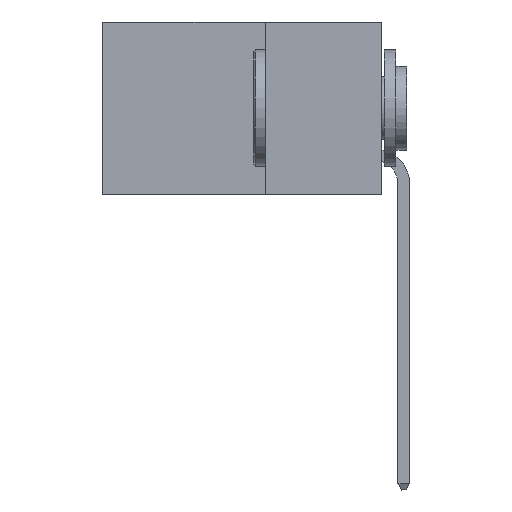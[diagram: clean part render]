
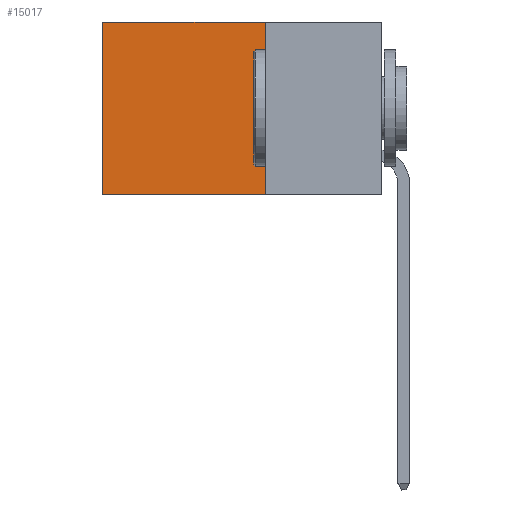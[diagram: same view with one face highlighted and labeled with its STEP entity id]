
A CAD part, left-side view. The second image highlights one B-rep face of the part: STEP entity #15017.
In plain terms, the highlighted planar face has unit normal (-1, 0, 0).
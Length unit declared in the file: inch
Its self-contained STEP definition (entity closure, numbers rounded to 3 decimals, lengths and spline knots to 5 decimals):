
#674 = LINE ( 'NONE', #44026, #37747 ) ;
#1916 = EDGE_LOOP ( 'NONE', ( #40481, #41834, #44903, #2438 ) ) ;
#2438 = ORIENTED_EDGE ( 'NONE', *, *, #30803, .T. ) ;
#5627 = DIRECTION ( 'NONE',  ( 0., 0., -1. ) ) ;
#7217 = EDGE_CURVE ( 'NONE', #43208, #20553, #37806, .T. ) ;
#10774 = VECTOR ( 'NONE', #5627, 39.37008 ) ;
#12456 = EDGE_CURVE ( 'NONE', #20553, #42299, #674, .T. ) ;
#13764 = CARTESIAN_POINT ( 'NONE',  ( 0.2875, 0.25, 0. ) ) ;
#14075 = DIRECTION ( 'NONE',  ( 0., 0., -1. ) ) ;
#14415 = VECTOR ( 'NONE', #17341, 39.37008 ) ;
#14515 = CARTESIAN_POINT ( 'NONE',  ( 0.2875, 0.25, 0. ) ) ;
#14993 = CARTESIAN_POINT ( 'NONE',  ( 0.2875, 0.25, -0.37 ) ) ;
#15017 = ADVANCED_FACE ( 'NONE', ( #31321 ), #45950, .F. ) ;
#17226 = CARTESIAN_POINT ( 'NONE',  ( 0.2875, 0.6, -0.37 ) ) ;
#17341 = DIRECTION ( 'NONE',  ( 0., 1., 0. ) ) ;
#19811 = CARTESIAN_POINT ( 'NONE',  ( 0.2875, 0.25, 0. ) ) ;
#20553 = VERTEX_POINT ( 'NONE', #14993 ) ;
#22053 = CARTESIAN_POINT ( 'NONE',  ( 0.2875, 0.6, 0. ) ) ;
#23967 = LINE ( 'NONE', #24135, #14415 ) ;
#24135 = CARTESIAN_POINT ( 'NONE',  ( 0.2875, 0.25, 0. ) ) ;
#26344 = DIRECTION ( 'NONE',  ( 0., 0., -1. ) ) ;
#29190 = DIRECTION ( 'NONE',  ( 0., 1., 0. ) ) ;
#29609 = EDGE_CURVE ( 'NONE', #32860, #42299, #34507, .T. ) ;
#30803 = EDGE_CURVE ( 'NONE', #43208, #32860, #23967, .T. ) ;
#31039 = AXIS2_PLACEMENT_3D ( 'NONE', #13764, #31911, #14075 ) ;
#31321 = FACE_OUTER_BOUND ( 'NONE', #1916, .T. ) ;
#31911 = DIRECTION ( 'NONE',  ( 1., 0., 0. ) ) ;
#32860 = VERTEX_POINT ( 'NONE', #22053 ) ;
#34507 = LINE ( 'NONE', #44476, #46339 ) ;
#37747 = VECTOR ( 'NONE', #29190, 39.37008 ) ;
#37806 = LINE ( 'NONE', #19811, #10774 ) ;
#40481 = ORIENTED_EDGE ( 'NONE', *, *, #29609, .T. ) ;
#41834 = ORIENTED_EDGE ( 'NONE', *, *, #12456, .F. ) ;
#42299 = VERTEX_POINT ( 'NONE', #17226 ) ;
#43208 = VERTEX_POINT ( 'NONE', #14515 ) ;
#44026 = CARTESIAN_POINT ( 'NONE',  ( 0.2875, 0.25, -0.37 ) ) ;
#44476 = CARTESIAN_POINT ( 'NONE',  ( 0.2875, 0.6, 0. ) ) ;
#44903 = ORIENTED_EDGE ( 'NONE', *, *, #7217, .F. ) ;
#45950 = PLANE ( 'NONE',  #31039 ) ;
#46339 = VECTOR ( 'NONE', #26344, 39.37008 ) ;
